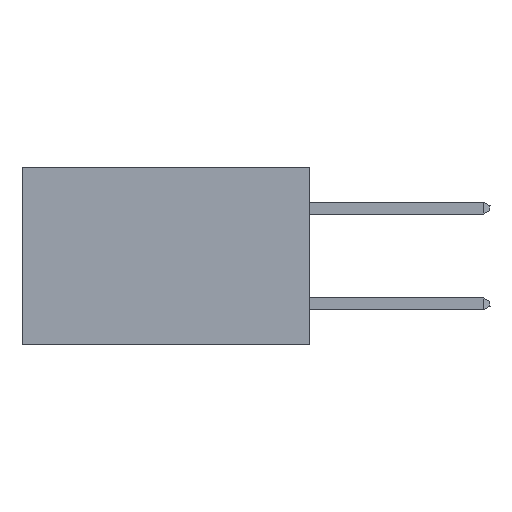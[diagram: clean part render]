
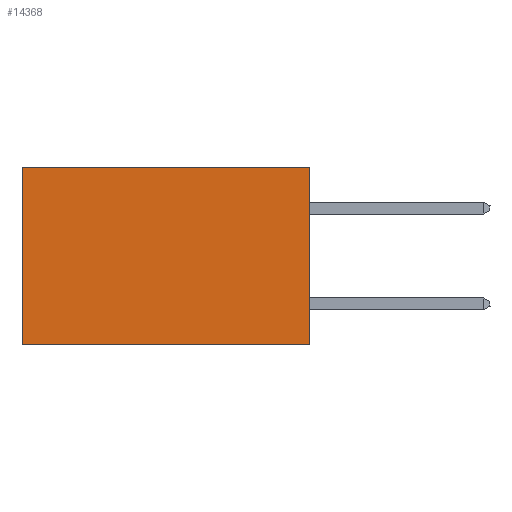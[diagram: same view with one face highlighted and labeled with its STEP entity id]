
A CAD part, left-side view. The second image highlights one B-rep face of the part: STEP entity #14368.
In plain terms, the highlighted planar face has unit normal (-1, 0, 0).
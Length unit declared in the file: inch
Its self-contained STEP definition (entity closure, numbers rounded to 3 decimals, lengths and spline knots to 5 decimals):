
#74 = FACE_OUTER_BOUND ( 'NONE', #7222, .T. ) ;
#114 = EDGE_CURVE ( 'NONE', #12994, #6768, #5770, .T. ) ;
#749 = CARTESIAN_POINT ( 'NONE',  ( 0.2875, 0., 0. ) ) ;
#1816 = CARTESIAN_POINT ( 'NONE',  ( 0.2875, 0.6, -0.37 ) ) ;
#2321 = DIRECTION ( 'NONE',  ( 0., 0., -1. ) ) ;
#2452 = PLANE ( 'NONE',  #2814 ) ;
#2814 = AXIS2_PLACEMENT_3D ( 'NONE', #13496, #14965, #5655 ) ;
#3747 = VECTOR ( 'NONE', #5417, 39.37008 ) ;
#4084 = VERTEX_POINT ( 'NONE', #10654 ) ;
#4346 = LINE ( 'NONE', #6690, #12228 ) ;
#5263 = VECTOR ( 'NONE', #17435, 39.37008 ) ;
#5417 = DIRECTION ( 'NONE',  ( 0., 1., 0. ) ) ;
#5655 = DIRECTION ( 'NONE',  ( 0., 0., -1. ) ) ;
#5770 = LINE ( 'NONE', #19159, #5263 ) ;
#6690 = CARTESIAN_POINT ( 'NONE',  ( 0.2875, 0.6, 0. ) ) ;
#6768 = VERTEX_POINT ( 'NONE', #11684 ) ;
#7222 = EDGE_LOOP ( 'NONE', ( #14856, #11914, #11165, #10847 ) ) ;
#8229 = EDGE_CURVE ( 'NONE', #4084, #15526, #19545, .T. ) ;
#8653 = CARTESIAN_POINT ( 'NONE',  ( 0.2875, 0., -0.37 ) ) ;
#8722 = LINE ( 'NONE', #749, #17367 ) ;
#9968 = DIRECTION ( 'NONE',  ( 0., 0., -1. ) ) ;
#10654 = CARTESIAN_POINT ( 'NONE',  ( 0.2875, 0., -0.37 ) ) ;
#10847 = ORIENTED_EDGE ( 'NONE', *, *, #114, .T. ) ;
#11165 = ORIENTED_EDGE ( 'NONE', *, *, #18517, .F. ) ;
#11684 = CARTESIAN_POINT ( 'NONE',  ( 0.2875, 0.6, 0. ) ) ;
#11914 = ORIENTED_EDGE ( 'NONE', *, *, #8229, .F. ) ;
#12228 = VECTOR ( 'NONE', #9968, 39.37008 ) ;
#12994 = VERTEX_POINT ( 'NONE', #16025 ) ;
#13062 = EDGE_CURVE ( 'NONE', #6768, #15526, #4346, .T. ) ;
#13496 = CARTESIAN_POINT ( 'NONE',  ( 0.2875, 0., 0. ) ) ;
#14368 = ADVANCED_FACE ( 'NONE', ( #74 ), #2452, .F. ) ;
#14856 = ORIENTED_EDGE ( 'NONE', *, *, #13062, .T. ) ;
#14965 = DIRECTION ( 'NONE',  ( 1., 0., 0. ) ) ;
#15526 = VERTEX_POINT ( 'NONE', #1816 ) ;
#16025 = CARTESIAN_POINT ( 'NONE',  ( 0.2875, 0., 0. ) ) ;
#17367 = VECTOR ( 'NONE', #2321, 39.37008 ) ;
#17435 = DIRECTION ( 'NONE',  ( 0., 1., 0. ) ) ;
#18517 = EDGE_CURVE ( 'NONE', #12994, #4084, #8722, .T. ) ;
#19159 = CARTESIAN_POINT ( 'NONE',  ( 0.2875, 0., 0. ) ) ;
#19545 = LINE ( 'NONE', #8653, #3747 ) ;
